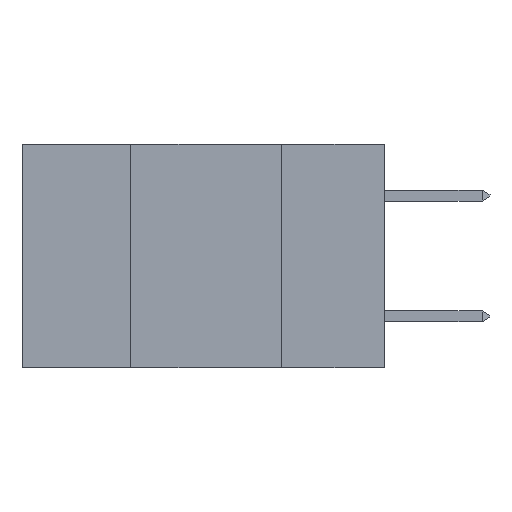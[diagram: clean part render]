
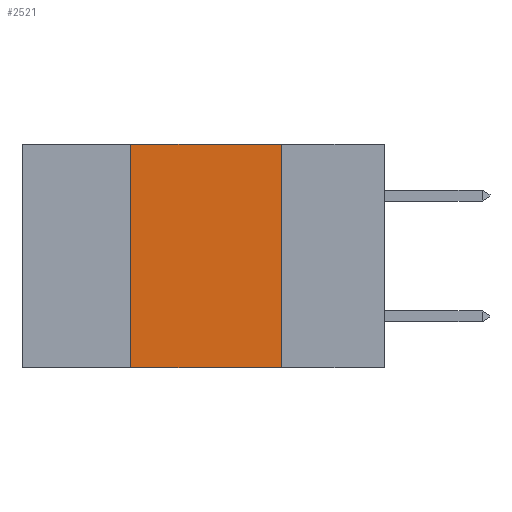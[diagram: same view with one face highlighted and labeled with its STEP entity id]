
A CAD part, left-side view. The second image highlights one B-rep face of the part: STEP entity #2521.
In plain terms, the highlighted planar face has unit normal (-1, 0, 0).
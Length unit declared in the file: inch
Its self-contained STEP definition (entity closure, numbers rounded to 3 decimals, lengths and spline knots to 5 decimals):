
#200 = VERTEX_POINT ( 'NONE', #3747 ) ;
#486 = EDGE_LOOP ( 'NONE', ( #8335, #8399, #8555, #8705 ) ) ;
#792 = CARTESIAN_POINT ( 'NONE',  ( 0., 0.6, 0. ) ) ;
#863 = VERTEX_POINT ( 'NONE', #3906 ) ;
#968 = EDGE_CURVE ( 'NONE', #863, #4006, #5583, .T. ) ;
#1626 = DIRECTION ( 'NONE',  ( 0., 0., -1. ) ) ;
#1751 = VECTOR ( 'NONE', #6892, 39.37008 ) ;
#2363 = LINE ( 'NONE', #4405, #4678 ) ;
#2521 = ADVANCED_FACE ( 'NONE', ( #10440 ), #10945, .F. ) ;
#3297 = VECTOR ( 'NONE', #5501, 39.37008 ) ;
#3747 = CARTESIAN_POINT ( 'NONE',  ( 0., 0.17, 0. ) ) ;
#3906 = CARTESIAN_POINT ( 'NONE',  ( 0., 0.42, -0.37 ) ) ;
#4006 = VERTEX_POINT ( 'NONE', #5378 ) ;
#4053 = LINE ( 'NONE', #7760, #1751 ) ;
#4057 = EDGE_CURVE ( 'NONE', #863, #7571, #4374, .T. ) ;
#4374 = LINE ( 'NONE', #7997, #10843 ) ;
#4405 = CARTESIAN_POINT ( 'NONE',  ( 0., 0.17, 0. ) ) ;
#4678 = VECTOR ( 'NONE', #8679, 39.37008 ) ;
#5378 = CARTESIAN_POINT ( 'NONE',  ( 0., 0.42, 0. ) ) ;
#5501 = DIRECTION ( 'NONE',  ( 0., 0., 1. ) ) ;
#5583 = LINE ( 'NONE', #8184, #3297 ) ;
#6149 = EDGE_CURVE ( 'NONE', #4006, #200, #4053, .T. ) ;
#6725 = AXIS2_PLACEMENT_3D ( 'NONE', #792, #9336, #1626 ) ;
#6892 = DIRECTION ( 'NONE',  ( 0., -1., 0. ) ) ;
#7571 = VERTEX_POINT ( 'NONE', #8751 ) ;
#7760 = CARTESIAN_POINT ( 'NONE',  ( 0., 0.6, 0. ) ) ;
#7997 = CARTESIAN_POINT ( 'NONE',  ( 0., 0.6, -0.37 ) ) ;
#8184 = CARTESIAN_POINT ( 'NONE',  ( 0., 0.42, 0. ) ) ;
#8335 = ORIENTED_EDGE ( 'NONE', *, *, #9596, .F. ) ;
#8399 = ORIENTED_EDGE ( 'NONE', *, *, #6149, .F. ) ;
#8555 = ORIENTED_EDGE ( 'NONE', *, *, #968, .F. ) ;
#8679 = DIRECTION ( 'NONE',  ( 0., 0., -1. ) ) ;
#8705 = ORIENTED_EDGE ( 'NONE', *, *, #4057, .T. ) ;
#8751 = CARTESIAN_POINT ( 'NONE',  ( 0., 0.17, -0.37 ) ) ;
#8865 = DIRECTION ( 'NONE',  ( 0., -1., 0. ) ) ;
#9336 = DIRECTION ( 'NONE',  ( 1., 0., 0. ) ) ;
#9596 = EDGE_CURVE ( 'NONE', #200, #7571, #2363, .T. ) ;
#10440 = FACE_OUTER_BOUND ( 'NONE', #486, .T. ) ;
#10843 = VECTOR ( 'NONE', #8865, 39.37008 ) ;
#10945 = PLANE ( 'NONE',  #6725 ) ;
